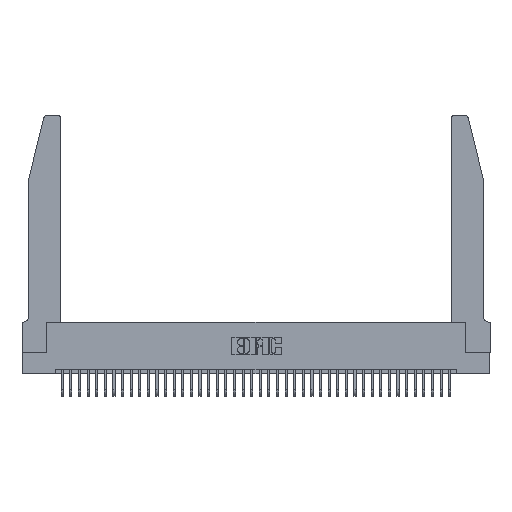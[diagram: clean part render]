
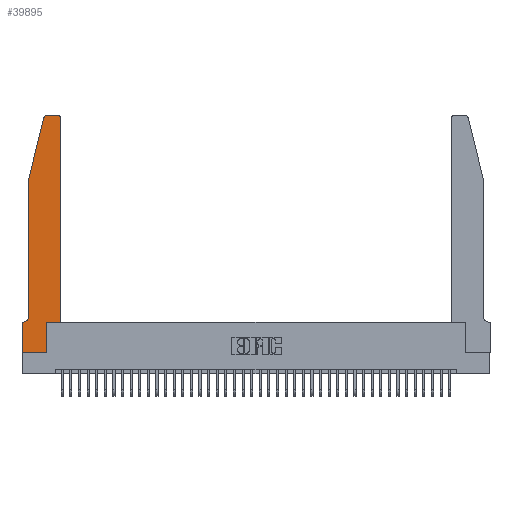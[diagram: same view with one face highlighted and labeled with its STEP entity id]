
A CAD part, top view. The second image highlights one B-rep face of the part: STEP entity #39895.
In plain terms, the highlighted planar face has unit normal (0, 0, 1).
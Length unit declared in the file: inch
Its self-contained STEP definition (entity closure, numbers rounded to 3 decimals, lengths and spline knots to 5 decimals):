
#537 = EDGE_CURVE ( 'NONE', #19994, #1420, #32093, .T. ) ;
#936 = ORIENTED_EDGE ( 'NONE', *, *, #37311, .T. ) ;
#958 = CARTESIAN_POINT ( 'NONE',  ( 0.0055, 0.42, 0.37 ) ) ;
#1324 = VERTEX_POINT ( 'NONE', #13298 ) ;
#1420 = VERTEX_POINT ( 'NONE', #25594 ) ;
#1747 = VECTOR ( 'NONE', #25252, 39.37008 ) ;
#2021 = LINE ( 'NONE', #8196, #17260 ) ;
#2066 = CARTESIAN_POINT ( 'NONE',  ( 0.0755, 2., 0.37 ) ) ;
#2231 = CIRCLE ( 'NONE', #17579, 0.07 ) ;
#3148 = VECTOR ( 'NONE', #11554, 39.37008 ) ;
#3994 = DIRECTION ( 'NONE',  ( -1., 0., 0. ) ) ;
#3996 = CIRCLE ( 'NONE', #40789, 0.03 ) ;
#4012 = ORIENTED_EDGE ( 'NONE', *, *, #21606, .T. ) ;
#5424 = PLANE ( 'NONE',  #37510 ) ;
#6049 = VERTEX_POINT ( 'NONE', #6857 ) ;
#6365 = LINE ( 'NONE', #26073, #19057 ) ;
#6648 = CIRCLE ( 'NONE', #23801, 0.03 ) ;
#6814 = VERTEX_POINT ( 'NONE', #7277 ) ;
#6857 = CARTESIAN_POINT ( 'NONE',  ( 0., 0., 0.37 ) ) ;
#7277 = CARTESIAN_POINT ( 'NONE',  ( 0.4205, 2.75, 0.37 ) ) ;
#7860 = CARTESIAN_POINT ( 'NONE',  ( 0.4205, 2.72, 0.37 ) ) ;
#8154 = CARTESIAN_POINT ( 'NONE',  ( 0.284, 2.72, 0.37 ) ) ;
#8196 = CARTESIAN_POINT ( 'NONE',  ( 0., 0., 0.37 ) ) ;
#9124 = VERTEX_POINT ( 'NONE', #23186 ) ;
#9385 = CARTESIAN_POINT ( 'NONE',  ( 0.0055, 0.35, 0.37 ) ) ;
#9748 = CARTESIAN_POINT ( 'NONE',  ( 0.0755, 2., 0.37 ) ) ;
#11554 = DIRECTION ( 'NONE',  ( -0.239, -0.971, 0. ) ) ;
#11604 = CARTESIAN_POINT ( 'NONE',  ( 0., 0.35, 0.37 ) ) ;
#12694 = LINE ( 'NONE', #16006, #16782 ) ;
#13298 = CARTESIAN_POINT ( 'NONE',  ( 0., 0.35, 0.37 ) ) ;
#14463 = VECTOR ( 'NONE', #33356, 39.37008 ) ;
#14581 = DIRECTION ( 'NONE',  ( 1., 0., 0. ) ) ;
#15187 = ORIENTED_EDGE ( 'NONE', *, *, #17172, .T. ) ;
#15620 = CARTESIAN_POINT ( 'NONE',  ( 0.2865, 0.35, 0.37 ) ) ;
#15950 = ORIENTED_EDGE ( 'NONE', *, *, #30020, .T. ) ;
#16006 = CARTESIAN_POINT ( 'NONE',  ( 0.0755, 0.35, 0.37 ) ) ;
#16193 = LINE ( 'NONE', #24684, #17641 ) ;
#16506 = ORIENTED_EDGE ( 'NONE', *, *, #32108, .T. ) ;
#16782 = VECTOR ( 'NONE', #38683, 39.37008 ) ;
#16836 = EDGE_CURVE ( 'NONE', #26840, #28630, #29388, .T. ) ;
#17172 = EDGE_CURVE ( 'NONE', #1420, #6814, #3996, .T. ) ;
#17260 = VECTOR ( 'NONE', #14581, 39.37008 ) ;
#17551 = LINE ( 'NONE', #22531, #14463 ) ;
#17579 = AXIS2_PLACEMENT_3D ( 'NONE', #958, #36167, #3994 ) ;
#17641 = VECTOR ( 'NONE', #37537, 39.37008 ) ;
#17788 = VERTEX_POINT ( 'NONE', #40754 ) ;
#18757 = CARTESIAN_POINT ( 'NONE',  ( 0.284, 2.75, 0.37 ) ) ;
#18768 = EDGE_CURVE ( 'NONE', #17788, #32068, #17551, .T. ) ;
#18769 = DIRECTION ( 'NONE',  ( 0., -1., 0. ) ) ;
#19057 = VECTOR ( 'NONE', #19452, 39.37008 ) ;
#19185 = ORIENTED_EDGE ( 'NONE', *, *, #22275, .T. ) ;
#19367 = CARTESIAN_POINT ( 'NONE',  ( 0.4505, 0.35, 0.37 ) ) ;
#19452 = DIRECTION ( 'NONE',  ( 1., 0., 0. ) ) ;
#19994 = VERTEX_POINT ( 'NONE', #19367 ) ;
#20101 = VERTEX_POINT ( 'NONE', #9385 ) ;
#21411 = LINE ( 'NONE', #2066, #3148 ) ;
#21606 = EDGE_CURVE ( 'NONE', #20101, #1324, #12694, .T. ) ;
#21709 = DIRECTION ( 'NONE',  ( 1., 0., 0. ) ) ;
#22185 = CARTESIAN_POINT ( 'NONE',  ( 0.0755, 2., 0.37 ) ) ;
#22275 = EDGE_CURVE ( 'NONE', #33797, #9124, #6648, .T. ) ;
#22531 = CARTESIAN_POINT ( 'NONE',  ( 0.2865, 0.35, 0.37 ) ) ;
#22998 = EDGE_LOOP ( 'NONE', ( #15950, #19185, #29573, #24981, #25809, #4012, #16506, #936, #25780, #31528, #40323, #15187 ) ) ;
#23116 = LINE ( 'NONE', #41400, #1747 ) ;
#23186 = CARTESIAN_POINT ( 'NONE',  ( 0.25487, 2.72718, 0.37 ) ) ;
#23427 = EDGE_CURVE ( 'NONE', #32068, #19994, #6365, .T. ) ;
#23724 = EDGE_CURVE ( 'NONE', #28630, #20101, #2231, .T. ) ;
#23801 = AXIS2_PLACEMENT_3D ( 'NONE', #8154, #34095, #34245 ) ;
#24339 = DIRECTION ( 'NONE',  ( 1., 0., 0. ) ) ;
#24684 = CARTESIAN_POINT ( 'NONE',  ( 0.2605, 2.75, 0.37 ) ) ;
#24981 = ORIENTED_EDGE ( 'NONE', *, *, #16836, .T. ) ;
#25252 = DIRECTION ( 'NONE',  ( 0., -1., 0. ) ) ;
#25594 = CARTESIAN_POINT ( 'NONE',  ( 0.4505, 2.72, 0.37 ) ) ;
#25780 = ORIENTED_EDGE ( 'NONE', *, *, #18768, .T. ) ;
#25809 = ORIENTED_EDGE ( 'NONE', *, *, #23724, .T. ) ;
#26073 = CARTESIAN_POINT ( 'NONE',  ( 0.4505, 0.35, 0.37 ) ) ;
#26840 = VERTEX_POINT ( 'NONE', #9748 ) ;
#28630 = VERTEX_POINT ( 'NONE', #34737 ) ;
#29388 = LINE ( 'NONE', #22185, #40003 ) ;
#29573 = ORIENTED_EDGE ( 'NONE', *, *, #35987, .T. ) ;
#30020 = EDGE_CURVE ( 'NONE', #6814, #33797, #16193, .T. ) ;
#30546 = DIRECTION ( 'NONE',  ( 0., 0., 1. ) ) ;
#31528 = ORIENTED_EDGE ( 'NONE', *, *, #23427, .T. ) ;
#32068 = VERTEX_POINT ( 'NONE', #15620 ) ;
#32093 = LINE ( 'NONE', #34651, #41739 ) ;
#32108 = EDGE_CURVE ( 'NONE', #1324, #6049, #23116, .T. ) ;
#33356 = DIRECTION ( 'NONE',  ( 0., 1., 0. ) ) ;
#33797 = VERTEX_POINT ( 'NONE', #18757 ) ;
#34095 = DIRECTION ( 'NONE',  ( 0., 0., 1. ) ) ;
#34147 = DIRECTION ( 'NONE',  ( 0., 0., 1. ) ) ;
#34245 = DIRECTION ( 'NONE',  ( 1., 0., 0. ) ) ;
#34651 = CARTESIAN_POINT ( 'NONE',  ( 0.4505, 0.35, 0.37 ) ) ;
#34737 = CARTESIAN_POINT ( 'NONE',  ( 0.0755, 0.42, 0.37 ) ) ;
#35987 = EDGE_CURVE ( 'NONE', #9124, #26840, #21411, .T. ) ;
#36167 = DIRECTION ( 'NONE',  ( 0., 0., -1. ) ) ;
#36313 = DIRECTION ( 'NONE',  ( 0., 1., 0. ) ) ;
#37311 = EDGE_CURVE ( 'NONE', #6049, #17788, #2021, .T. ) ;
#37510 = AXIS2_PLACEMENT_3D ( 'NONE', #11604, #34147, #21709 ) ;
#37537 = DIRECTION ( 'NONE',  ( -1., 0., 0. ) ) ;
#38683 = DIRECTION ( 'NONE',  ( -1., 0., 0. ) ) ;
#39895 = ADVANCED_FACE ( 'NONE', ( #40393 ), #5424, .T. ) ;
#40003 = VECTOR ( 'NONE', #18769, 39.37008 ) ;
#40323 = ORIENTED_EDGE ( 'NONE', *, *, #537, .T. ) ;
#40393 = FACE_OUTER_BOUND ( 'NONE', #22998, .T. ) ;
#40754 = CARTESIAN_POINT ( 'NONE',  ( 0.2865, 0., 0.37 ) ) ;
#40789 = AXIS2_PLACEMENT_3D ( 'NONE', #7860, #30546, #24339 ) ;
#41400 = CARTESIAN_POINT ( 'NONE',  ( 0., 0., 0.37 ) ) ;
#41739 = VECTOR ( 'NONE', #36313, 39.37008 ) ;
